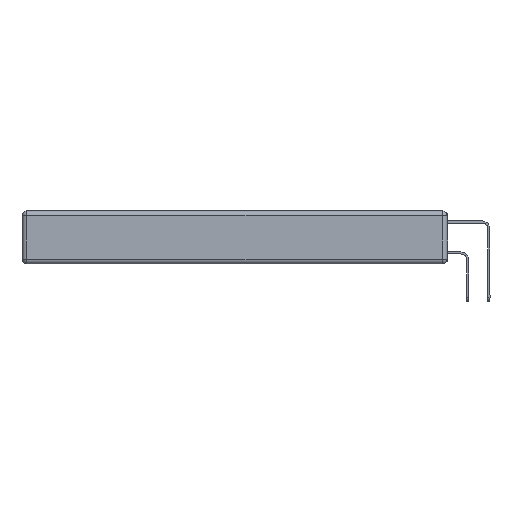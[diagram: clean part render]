
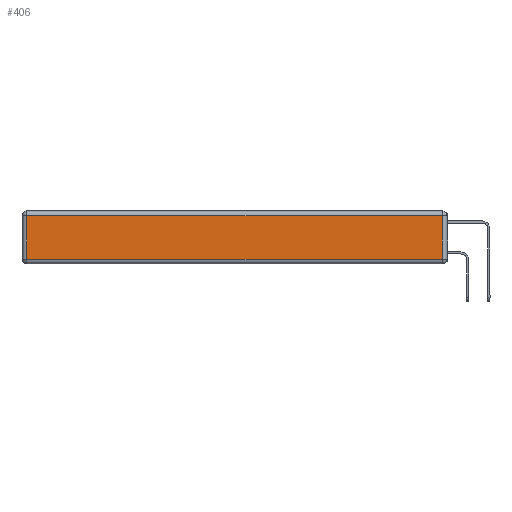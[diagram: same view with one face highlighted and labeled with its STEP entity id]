
A CAD part, left-side view. The second image highlights one B-rep face of the part: STEP entity #406.
In plain terms, the highlighted planar face has unit normal (-1, 0, 0).
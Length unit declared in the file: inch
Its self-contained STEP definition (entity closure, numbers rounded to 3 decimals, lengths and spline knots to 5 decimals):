
#406 = ADVANCED_FACE ( 'NONE', ( #16856 ), #8910, .T. ) ;
#743 = ORIENTED_EDGE ( 'NONE', *, *, #14148, .T. ) ;
#1133 = CARTESIAN_POINT ( 'NONE',  ( 0., 0.03, -0.343 ) ) ;
#1541 = AXIS2_PLACEMENT_3D ( 'NONE', #14176, #2346, #16936 ) ;
#1896 = ORIENTED_EDGE ( 'NONE', *, *, #11719, .T. ) ;
#2000 = EDGE_CURVE ( 'NONE', #5060, #5504, #3418, .T. ) ;
#2159 = LINE ( 'NONE', #16483, #11967 ) ;
#2346 = DIRECTION ( 'NONE',  ( -1., 0., 0. ) ) ;
#3418 = LINE ( 'NONE', #8675, #11794 ) ;
#5060 = VERTEX_POINT ( 'NONE', #13982 ) ;
#5336 = EDGE_CURVE ( 'NONE', #5504, #8769, #6900, .T. ) ;
#5504 = VERTEX_POINT ( 'NONE', #16383 ) ;
#6900 = LINE ( 'NONE', #7065, #7183 ) ;
#7065 = CARTESIAN_POINT ( 'NONE',  ( 0., 2.72, -0.343 ) ) ;
#7183 = VECTOR ( 'NONE', #10671, 39.37008 ) ;
#8675 = CARTESIAN_POINT ( 'NONE',  ( 0., 2.75, -0.03 ) ) ;
#8769 = VERTEX_POINT ( 'NONE', #12287 ) ;
#8865 = CARTESIAN_POINT ( 'NONE',  ( 0., 0.03, -0.313 ) ) ;
#8910 = PLANE ( 'NONE',  #1541 ) ;
#10671 = DIRECTION ( 'NONE',  ( 0., 0., -1. ) ) ;
#11577 = DIRECTION ( 'NONE',  ( 0., 0., 1. ) ) ;
#11719 = EDGE_CURVE ( 'NONE', #8769, #13246, #2159, .T. ) ;
#11794 = VECTOR ( 'NONE', #13940, 39.37008 ) ;
#11967 = VECTOR ( 'NONE', #15188, 39.37008 ) ;
#12154 = EDGE_LOOP ( 'NONE', ( #1896, #743, #17048, #14273 ) ) ;
#12287 = CARTESIAN_POINT ( 'NONE',  ( 0., 2.72, -0.313 ) ) ;
#12631 = LINE ( 'NONE', #1133, #14010 ) ;
#13246 = VERTEX_POINT ( 'NONE', #8865 ) ;
#13940 = DIRECTION ( 'NONE',  ( 0., 1., 0. ) ) ;
#13982 = CARTESIAN_POINT ( 'NONE',  ( 0., 0.03, -0.03 ) ) ;
#14010 = VECTOR ( 'NONE', #11577, 39.37008 ) ;
#14148 = EDGE_CURVE ( 'NONE', #13246, #5060, #12631, .T. ) ;
#14176 = CARTESIAN_POINT ( 'NONE',  ( 0., 0., -0.343 ) ) ;
#14273 = ORIENTED_EDGE ( 'NONE', *, *, #5336, .T. ) ;
#15188 = DIRECTION ( 'NONE',  ( 0., -1., 0. ) ) ;
#16383 = CARTESIAN_POINT ( 'NONE',  ( 0., 2.72, -0.03 ) ) ;
#16483 = CARTESIAN_POINT ( 'NONE',  ( 0., 0., -0.313 ) ) ;
#16856 = FACE_OUTER_BOUND ( 'NONE', #12154, .T. ) ;
#16936 = DIRECTION ( 'NONE',  ( 0., 0., 1. ) ) ;
#17048 = ORIENTED_EDGE ( 'NONE', *, *, #2000, .T. ) ;
